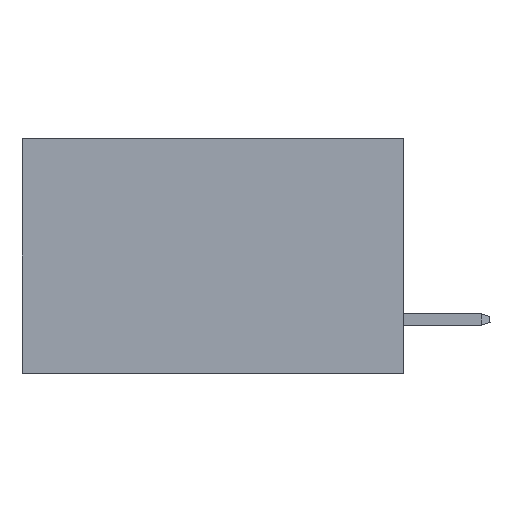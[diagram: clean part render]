
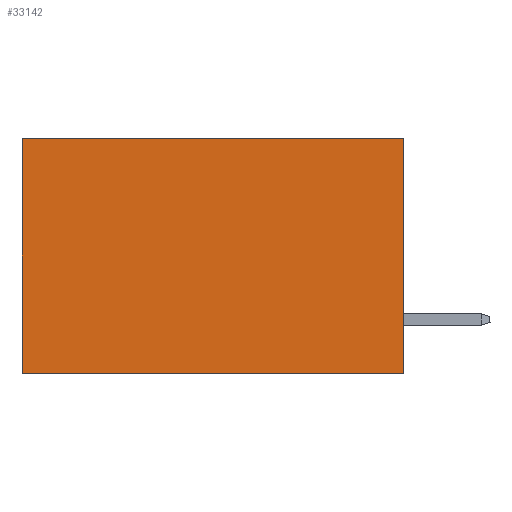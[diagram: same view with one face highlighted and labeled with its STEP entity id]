
A CAD part, left-side view. The second image highlights one B-rep face of the part: STEP entity #33142.
In plain terms, the highlighted planar face has unit normal (-1, 0, 0).
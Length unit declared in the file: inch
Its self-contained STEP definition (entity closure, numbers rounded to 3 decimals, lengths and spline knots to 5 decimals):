
#41 = CARTESIAN_POINT ( 'NONE',  ( 0.2875, 0., 0. ) ) ;
#1460 = DIRECTION ( 'NONE',  ( 0., 0., -1. ) ) ;
#1970 = CARTESIAN_POINT ( 'NONE',  ( 0.2875, 0., 0. ) ) ;
#2960 = LINE ( 'NONE', #41, #22948 ) ;
#2990 = ORIENTED_EDGE ( 'NONE', *, *, #20665, .F. ) ;
#3424 = VERTEX_POINT ( 'NONE', #18012 ) ;
#3616 = LINE ( 'NONE', #8755, #30847 ) ;
#4049 = VERTEX_POINT ( 'NONE', #23790 ) ;
#4309 = CARTESIAN_POINT ( 'NONE',  ( 0.2875, 0., 0. ) ) ;
#5990 = ORIENTED_EDGE ( 'NONE', *, *, #9739, .T. ) ;
#7115 = LINE ( 'NONE', #1970, #31228 ) ;
#8141 = LINE ( 'NONE', #8486, #20596 ) ;
#8486 = CARTESIAN_POINT ( 'NONE',  ( 0.2875, 0., -0.37 ) ) ;
#8755 = CARTESIAN_POINT ( 'NONE',  ( 0.2875, 0.6, 0. ) ) ;
#9291 = EDGE_LOOP ( 'NONE', ( #32719, #17825, #2990, #5990 ) ) ;
#9392 = EDGE_CURVE ( 'NONE', #33713, #3424, #8141, .T. ) ;
#9739 = EDGE_CURVE ( 'NONE', #17146, #4049, #2960, .T. ) ;
#14330 = AXIS2_PLACEMENT_3D ( 'NONE', #20276, #17875, #22510 ) ;
#17146 = VERTEX_POINT ( 'NONE', #4309 ) ;
#17825 = ORIENTED_EDGE ( 'NONE', *, *, #9392, .F. ) ;
#17875 = DIRECTION ( 'NONE',  ( 1., 0., 0. ) ) ;
#18012 = CARTESIAN_POINT ( 'NONE',  ( 0.2875, 0.6, -0.37 ) ) ;
#18757 = DIRECTION ( 'NONE',  ( 0., 1., 0. ) ) ;
#19029 = DIRECTION ( 'NONE',  ( 0., 0., -1. ) ) ;
#20276 = CARTESIAN_POINT ( 'NONE',  ( 0.2875, 0., 0. ) ) ;
#20596 = VECTOR ( 'NONE', #18757, 39.37008 ) ;
#20665 = EDGE_CURVE ( 'NONE', #17146, #33713, #7115, .T. ) ;
#22510 = DIRECTION ( 'NONE',  ( 0., 0., -1. ) ) ;
#22948 = VECTOR ( 'NONE', #26246, 39.37008 ) ;
#23790 = CARTESIAN_POINT ( 'NONE',  ( 0.2875, 0.6, 0. ) ) ;
#24601 = EDGE_CURVE ( 'NONE', #4049, #3424, #3616, .T. ) ;
#26246 = DIRECTION ( 'NONE',  ( 0., 1., 0. ) ) ;
#28162 = FACE_OUTER_BOUND ( 'NONE', #9291, .T. ) ;
#29433 = CARTESIAN_POINT ( 'NONE',  ( 0.2875, 0., -0.37 ) ) ;
#30743 = PLANE ( 'NONE',  #14330 ) ;
#30847 = VECTOR ( 'NONE', #19029, 39.37008 ) ;
#31228 = VECTOR ( 'NONE', #1460, 39.37008 ) ;
#32719 = ORIENTED_EDGE ( 'NONE', *, *, #24601, .T. ) ;
#33142 = ADVANCED_FACE ( 'NONE', ( #28162 ), #30743, .F. ) ;
#33713 = VERTEX_POINT ( 'NONE', #29433 ) ;
